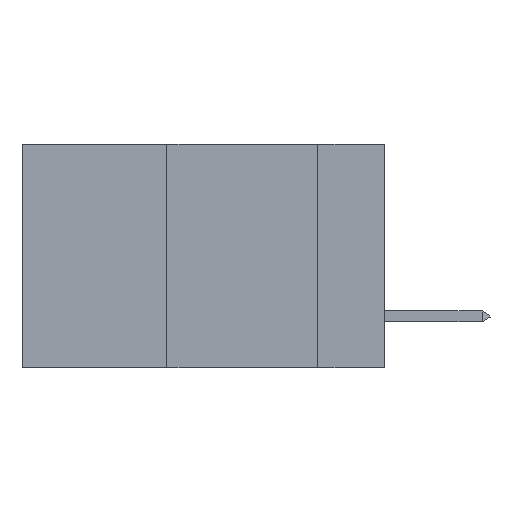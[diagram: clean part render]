
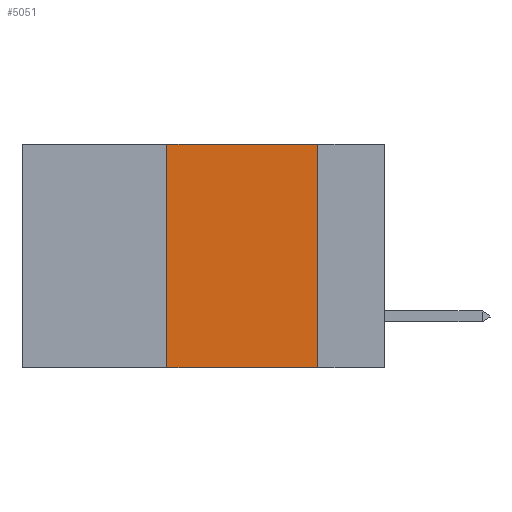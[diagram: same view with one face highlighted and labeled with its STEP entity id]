
A CAD part, left-side view. The second image highlights one B-rep face of the part: STEP entity #5051.
In plain terms, the highlighted planar face has unit normal (-1, 0, 0).
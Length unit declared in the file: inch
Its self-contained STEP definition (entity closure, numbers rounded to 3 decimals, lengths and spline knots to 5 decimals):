
#646 = ORIENTED_EDGE ( 'NONE', *, *, #28391, .F. ) ;
#701 = VECTOR ( 'NONE', #24116, 39.37008 ) ;
#1877 = ORIENTED_EDGE ( 'NONE', *, *, #12724, .F. ) ;
#3549 = CARTESIAN_POINT ( 'NONE',  ( 0., 0.36, 0. ) ) ;
#4160 = LINE ( 'NONE', #14948, #701 ) ;
#5051 = ADVANCED_FACE ( 'NONE', ( #16279 ), #11327, .F. ) ;
#7412 = CARTESIAN_POINT ( 'NONE',  ( 0., 0.11, 0. ) ) ;
#8575 = EDGE_LOOP ( 'NONE', ( #646, #1877, #33930, #18370 ) ) ;
#9692 = VERTEX_POINT ( 'NONE', #39652 ) ;
#11327 = PLANE ( 'NONE',  #30289 ) ;
#12654 = VERTEX_POINT ( 'NONE', #19648 ) ;
#12724 = EDGE_CURVE ( 'NONE', #20082, #38901, #4160, .T. ) ;
#13381 = CARTESIAN_POINT ( 'NONE',  ( 0., 0.36, 0. ) ) ;
#13934 = VECTOR ( 'NONE', #28786, 39.37008 ) ;
#14011 = LINE ( 'NONE', #3549, #34408 ) ;
#14948 = CARTESIAN_POINT ( 'NONE',  ( 0., 0.6, 0. ) ) ;
#16279 = FACE_OUTER_BOUND ( 'NONE', #8575, .T. ) ;
#16460 = DIRECTION ( 'NONE',  ( 0., 0., 1. ) ) ;
#18370 = ORIENTED_EDGE ( 'NONE', *, *, #38788, .T. ) ;
#19315 = CARTESIAN_POINT ( 'NONE',  ( 0., 0.11, 0. ) ) ;
#19648 = CARTESIAN_POINT ( 'NONE',  ( 0., 0.11, -0.37 ) ) ;
#20082 = VERTEX_POINT ( 'NONE', #13381 ) ;
#22377 = LINE ( 'NONE', #19315, #13934 ) ;
#22556 = DIRECTION ( 'NONE',  ( 0., -1., 0. ) ) ;
#23939 = VECTOR ( 'NONE', #22556, 39.37008 ) ;
#24116 = DIRECTION ( 'NONE',  ( 0., -1., 0. ) ) ;
#24258 = CARTESIAN_POINT ( 'NONE',  ( 0., 0.6, 0. ) ) ;
#27365 = EDGE_CURVE ( 'NONE', #9692, #20082, #14011, .T. ) ;
#28391 = EDGE_CURVE ( 'NONE', #38901, #12654, #22377, .T. ) ;
#28680 = CARTESIAN_POINT ( 'NONE',  ( 0., 0.6, -0.37 ) ) ;
#28786 = DIRECTION ( 'NONE',  ( 0., 0., -1. ) ) ;
#30289 = AXIS2_PLACEMENT_3D ( 'NONE', #24258, #40021, #36978 ) ;
#31348 = LINE ( 'NONE', #28680, #23939 ) ;
#33930 = ORIENTED_EDGE ( 'NONE', *, *, #27365, .F. ) ;
#34408 = VECTOR ( 'NONE', #16460, 39.37008 ) ;
#36978 = DIRECTION ( 'NONE',  ( 0., 0., -1. ) ) ;
#38788 = EDGE_CURVE ( 'NONE', #9692, #12654, #31348, .T. ) ;
#38901 = VERTEX_POINT ( 'NONE', #7412 ) ;
#39652 = CARTESIAN_POINT ( 'NONE',  ( 0., 0.36, -0.37 ) ) ;
#40021 = DIRECTION ( 'NONE',  ( 1., 0., 0. ) ) ;
